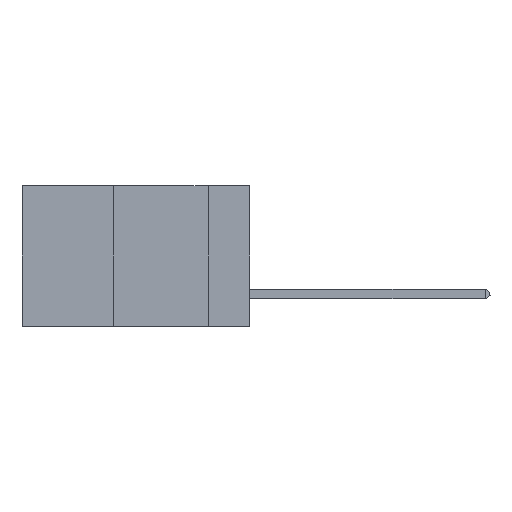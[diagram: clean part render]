
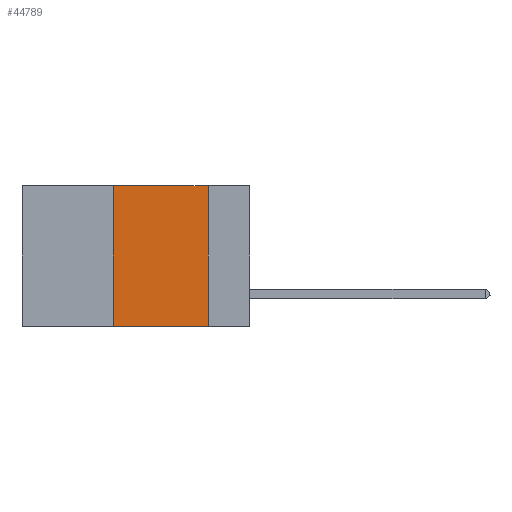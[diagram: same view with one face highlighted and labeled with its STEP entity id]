
A CAD part, left-side view. The second image highlights one B-rep face of the part: STEP entity #44789.
In plain terms, the highlighted planar face has unit normal (-1, 0, 0).
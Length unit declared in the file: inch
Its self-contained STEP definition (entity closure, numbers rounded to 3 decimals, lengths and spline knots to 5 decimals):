
#140 = CARTESIAN_POINT ( 'NONE',  ( 0., 0.36, 0. ) ) ;
#820 = CARTESIAN_POINT ( 'NONE',  ( 0., 0.6, 0. ) ) ;
#2393 = VECTOR ( 'NONE', #34490, 39.37008 ) ;
#2862 = PLANE ( 'NONE',  #3456 ) ;
#2889 = CARTESIAN_POINT ( 'NONE',  ( 0., 0.11, -0.37 ) ) ;
#3456 = AXIS2_PLACEMENT_3D ( 'NONE', #11121, #22213, #30048 ) ;
#6320 = EDGE_LOOP ( 'NONE', ( #21441, #15980, #20082, #18268 ) ) ;
#6461 = EDGE_CURVE ( 'NONE', #13097, #45392, #35728, .T. ) ;
#7920 = DIRECTION ( 'NONE',  ( 0., 0., 1. ) ) ;
#9232 = CARTESIAN_POINT ( 'NONE',  ( 0., 0.11, 0. ) ) ;
#10098 = VECTOR ( 'NONE', #46477, 39.37008 ) ;
#11121 = CARTESIAN_POINT ( 'NONE',  ( 0., 0.6, 0. ) ) ;
#11160 = CARTESIAN_POINT ( 'NONE',  ( 0., 0.6, -0.37 ) ) ;
#11214 = VERTEX_POINT ( 'NONE', #9232 ) ;
#13097 = VERTEX_POINT ( 'NONE', #21950 ) ;
#14972 = LINE ( 'NONE', #18337, #35649 ) ;
#15980 = ORIENTED_EDGE ( 'NONE', *, *, #33088, .F. ) ;
#16259 = VECTOR ( 'NONE', #7920, 39.37008 ) ;
#18268 = ORIENTED_EDGE ( 'NONE', *, *, #44285, .T. ) ;
#18337 = CARTESIAN_POINT ( 'NONE',  ( 0., 0.11, 0. ) ) ;
#20082 = ORIENTED_EDGE ( 'NONE', *, *, #6461, .F. ) ;
#21441 = ORIENTED_EDGE ( 'NONE', *, *, #46039, .F. ) ;
#21950 = CARTESIAN_POINT ( 'NONE',  ( 0., 0.36, -0.37 ) ) ;
#22213 = DIRECTION ( 'NONE',  ( 1., 0., 0. ) ) ;
#22322 = CARTESIAN_POINT ( 'NONE',  ( 0., 0.36, 0. ) ) ;
#24091 = VERTEX_POINT ( 'NONE', #2889 ) ;
#25377 = LINE ( 'NONE', #820, #10098 ) ;
#30048 = DIRECTION ( 'NONE',  ( 0., 0., -1. ) ) ;
#33088 = EDGE_CURVE ( 'NONE', #45392, #11214, #25377, .T. ) ;
#33983 = DIRECTION ( 'NONE',  ( 0., 0., -1. ) ) ;
#34490 = DIRECTION ( 'NONE',  ( 0., -1., 0. ) ) ;
#35649 = VECTOR ( 'NONE', #33983, 39.37008 ) ;
#35728 = LINE ( 'NONE', #140, #16259 ) ;
#37577 = FACE_OUTER_BOUND ( 'NONE', #6320, .T. ) ;
#44285 = EDGE_CURVE ( 'NONE', #13097, #24091, #49742, .T. ) ;
#44789 = ADVANCED_FACE ( 'NONE', ( #37577 ), #2862, .F. ) ;
#45392 = VERTEX_POINT ( 'NONE', #22322 ) ;
#46039 = EDGE_CURVE ( 'NONE', #11214, #24091, #14972, .T. ) ;
#46477 = DIRECTION ( 'NONE',  ( 0., -1., 0. ) ) ;
#49742 = LINE ( 'NONE', #11160, #2393 ) ;
